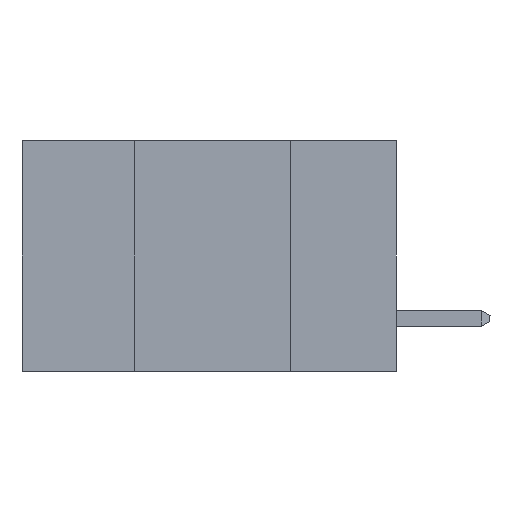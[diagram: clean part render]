
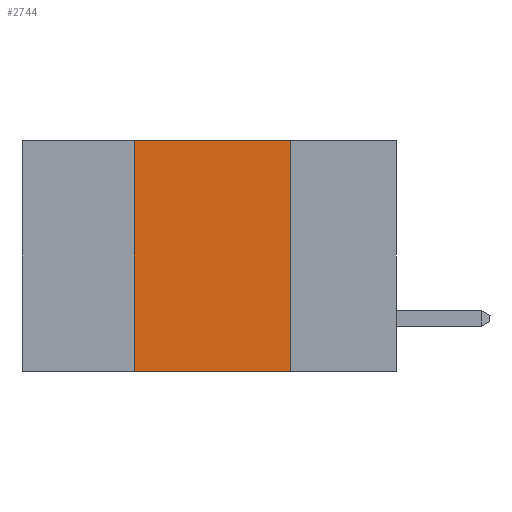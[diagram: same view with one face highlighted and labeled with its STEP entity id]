
A CAD part, left-side view. The second image highlights one B-rep face of the part: STEP entity #2744.
In plain terms, the highlighted planar face has unit normal (-1, 0, 0).
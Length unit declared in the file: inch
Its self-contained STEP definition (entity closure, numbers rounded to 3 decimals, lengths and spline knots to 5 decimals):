
#1142 = VERTEX_POINT ( 'NONE', #14571 ) ;
#1312 = EDGE_CURVE ( 'NONE', #9588, #7394, #3138, .T. ) ;
#2289 = DIRECTION ( 'NONE',  ( 1., 0., 0. ) ) ;
#2744 = ADVANCED_FACE ( 'NONE', ( #7302 ), #14434, .F. ) ;
#3103 = LINE ( 'NONE', #4068, #7062 ) ;
#3138 = LINE ( 'NONE', #4345, #10028 ) ;
#3205 = LINE ( 'NONE', #5440, #12115 ) ;
#3318 = ORIENTED_EDGE ( 'NONE', *, *, #5645, .T. ) ;
#4068 = CARTESIAN_POINT ( 'NONE',  ( 0., 0.6, -0.37 ) ) ;
#4345 = CARTESIAN_POINT ( 'NONE',  ( 0., 0.6, 0. ) ) ;
#4675 = LINE ( 'NONE', #12263, #9447 ) ;
#4908 = CARTESIAN_POINT ( 'NONE',  ( 0., 0.6, 0. ) ) ;
#5148 = CARTESIAN_POINT ( 'NONE',  ( 0., 0.42, -0.37 ) ) ;
#5440 = CARTESIAN_POINT ( 'NONE',  ( 0., 0.17, -0.37 ) ) ;
#5525 = DIRECTION ( 'NONE',  ( 0., -1., 0. ) ) ;
#5645 = EDGE_CURVE ( 'NONE', #13838, #1142, #3103, .T. ) ;
#7062 = VECTOR ( 'NONE', #8910, 39.37008 ) ;
#7074 = DIRECTION ( 'NONE',  ( 0., 0., -1. ) ) ;
#7302 = FACE_OUTER_BOUND ( 'NONE', #9972, .T. ) ;
#7394 = VERTEX_POINT ( 'NONE', #11432 ) ;
#8848 = ORIENTED_EDGE ( 'NONE', *, *, #1312, .F. ) ;
#8910 = DIRECTION ( 'NONE',  ( 0., -1., 0. ) ) ;
#9447 = VECTOR ( 'NONE', #11004, 39.37008 ) ;
#9588 = VERTEX_POINT ( 'NONE', #10365 ) ;
#9972 = EDGE_LOOP ( 'NONE', ( #12013, #8848, #13646, #3318 ) ) ;
#10028 = VECTOR ( 'NONE', #5525, 39.37008 ) ;
#10365 = CARTESIAN_POINT ( 'NONE',  ( 0., 0.42, 0. ) ) ;
#11004 = DIRECTION ( 'NONE',  ( 0., 0., 1. ) ) ;
#11432 = CARTESIAN_POINT ( 'NONE',  ( 0., 0.17, 0. ) ) ;
#11434 = EDGE_CURVE ( 'NONE', #7394, #1142, #3205, .T. ) ;
#12013 = ORIENTED_EDGE ( 'NONE', *, *, #11434, .F. ) ;
#12115 = VECTOR ( 'NONE', #12746, 39.37008 ) ;
#12263 = CARTESIAN_POINT ( 'NONE',  ( 0., 0.42, -0.37 ) ) ;
#12328 = AXIS2_PLACEMENT_3D ( 'NONE', #4908, #2289, #7074 ) ;
#12746 = DIRECTION ( 'NONE',  ( 0., 0., -1. ) ) ;
#13646 = ORIENTED_EDGE ( 'NONE', *, *, #14397, .F. ) ;
#13838 = VERTEX_POINT ( 'NONE', #5148 ) ;
#14397 = EDGE_CURVE ( 'NONE', #13838, #9588, #4675, .T. ) ;
#14434 = PLANE ( 'NONE',  #12328 ) ;
#14571 = CARTESIAN_POINT ( 'NONE',  ( 0., 0.17, -0.37 ) ) ;
